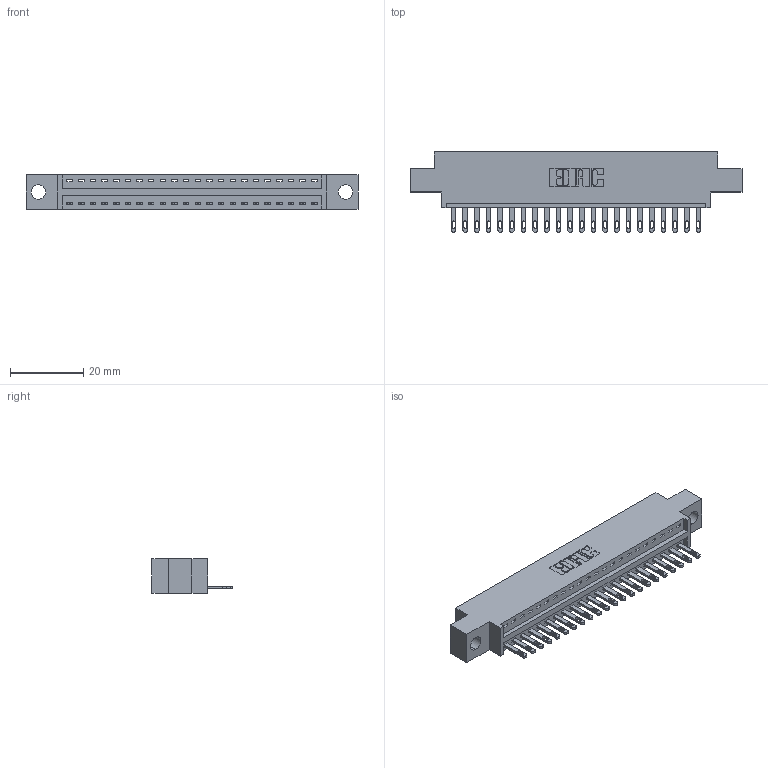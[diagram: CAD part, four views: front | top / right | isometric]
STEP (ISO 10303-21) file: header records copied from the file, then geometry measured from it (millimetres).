
FILE_DESCRIPTION (( 'STEP AP203' ), '1' );
FILE_NAME ('346-022-500-604.STEP', '2018-08-20T23:32:49', ( '' ), ( '' ), 'SwSTEP 2.0', 'SolidWorks 2016', '' );
FILE_SCHEMA (( 'CONFIG_CONTROL_DESIGN' ));
Length unit declared in the file: inch
Products named in the file (3): 345-292-001_345-293-100; 346-022-500-604; 346 Part_0.170 Offset - 0.156 Dia-TH
Assembly tree (23 placements, depth 2):
  346-022-500-604
    346 Part_0.170 Offset - 0.156 Dia-TH
    345-292-001_345-293-100  x22
Bounding box: 90.42 x 21.84 x 9.4 mm (x, y, z)
Volume: 8288.9 mm3; surface area: 10160.8 mm2
Topology: 23 solids, 23 shells, 1314 faces, 4037 edges, 2690 vertices
Faces by surface type: plane 828, cylinder 486
Entity records: 16411 total; most frequent: CARTESIAN_POINT 2826, ORIENTED_EDGE 2782, DIRECTION 2519, EDGE_CURVE 1391, VECTOR 1167, LINE 1167, VERTEX_POINT 926, AXIS2_PLACEMENT_3D 676
